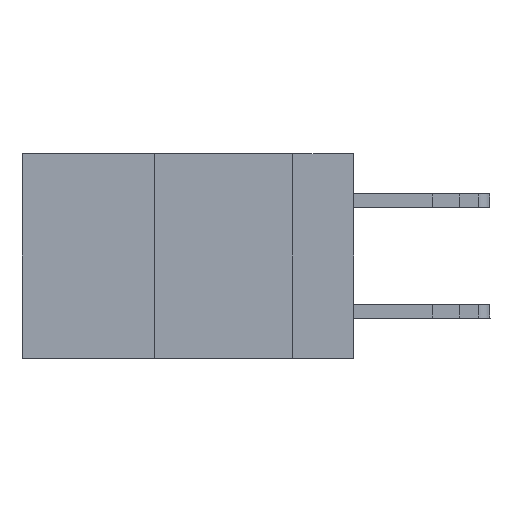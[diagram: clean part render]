
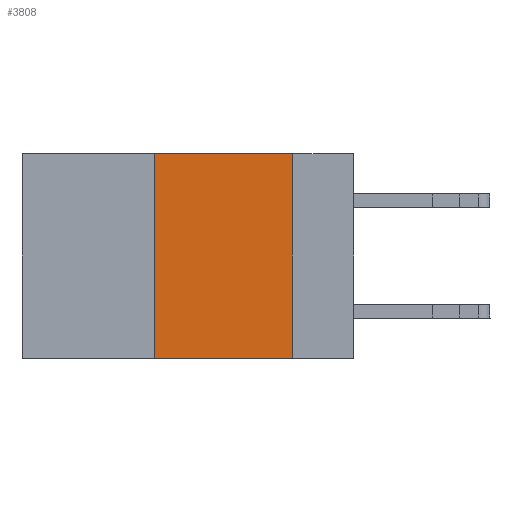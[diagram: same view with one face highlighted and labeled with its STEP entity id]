
A CAD part, left-side view. The second image highlights one B-rep face of the part: STEP entity #3808.
In plain terms, the highlighted planar face has unit normal (-1, 0, 0).
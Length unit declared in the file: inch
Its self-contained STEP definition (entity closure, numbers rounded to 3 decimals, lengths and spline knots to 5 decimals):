
#539 = FACE_OUTER_BOUND ( 'NONE', #1060, .T. ) ;
#824 = CARTESIAN_POINT ( 'NONE',  ( 0., 0.11, -0.37 ) ) ;
#966 = AXIS2_PLACEMENT_3D ( 'NONE', #1714, #16997, #7418 ) ;
#981 = VERTEX_POINT ( 'NONE', #6675 ) ;
#1012 = ORIENTED_EDGE ( 'NONE', *, *, #10371, .F. ) ;
#1060 = EDGE_LOOP ( 'NONE', ( #17634, #1012, #13462, #4346 ) ) ;
#1296 = LINE ( 'NONE', #4005, #12722 ) ;
#1714 = CARTESIAN_POINT ( 'NONE',  ( 0., 0.6, 0. ) ) ;
#2672 = DIRECTION ( 'NONE',  ( 0., -1., 0. ) ) ;
#2732 = EDGE_CURVE ( 'NONE', #981, #13722, #12860, .T. ) ;
#3287 = VECTOR ( 'NONE', #2672, 39.37008 ) ;
#3808 = ADVANCED_FACE ( 'NONE', ( #539 ), #10044, .F. ) ;
#4005 = CARTESIAN_POINT ( 'NONE',  ( 0., 0.11, 0. ) ) ;
#4219 = VERTEX_POINT ( 'NONE', #14077 ) ;
#4346 = ORIENTED_EDGE ( 'NONE', *, *, #14621, .T. ) ;
#5191 = LINE ( 'NONE', #17231, #6292 ) ;
#5352 = VERTEX_POINT ( 'NONE', #824 ) ;
#5564 = CARTESIAN_POINT ( 'NONE',  ( 0., 0.6, 0. ) ) ;
#6292 = VECTOR ( 'NONE', #9259, 39.37008 ) ;
#6675 = CARTESIAN_POINT ( 'NONE',  ( 0., 0.36, -0.37 ) ) ;
#7063 = CARTESIAN_POINT ( 'NONE',  ( 0., 0.36, 0. ) ) ;
#7418 = DIRECTION ( 'NONE',  ( 0., 0., -1. ) ) ;
#7817 = EDGE_CURVE ( 'NONE', #4219, #5352, #1296, .T. ) ;
#7864 = CARTESIAN_POINT ( 'NONE',  ( 0., 0.36, 0. ) ) ;
#8353 = DIRECTION ( 'NONE',  ( 0., 0., -1. ) ) ;
#9259 = DIRECTION ( 'NONE',  ( 0., -1., 0. ) ) ;
#10044 = PLANE ( 'NONE',  #966 ) ;
#10371 = EDGE_CURVE ( 'NONE', #13722, #4219, #12105, .T. ) ;
#10564 = VECTOR ( 'NONE', #12948, 39.37008 ) ;
#12105 = LINE ( 'NONE', #5564, #3287 ) ;
#12722 = VECTOR ( 'NONE', #8353, 39.37008 ) ;
#12860 = LINE ( 'NONE', #7063, #10564 ) ;
#12948 = DIRECTION ( 'NONE',  ( 0., 0., 1. ) ) ;
#13462 = ORIENTED_EDGE ( 'NONE', *, *, #2732, .F. ) ;
#13722 = VERTEX_POINT ( 'NONE', #7864 ) ;
#14077 = CARTESIAN_POINT ( 'NONE',  ( 0., 0.11, 0. ) ) ;
#14621 = EDGE_CURVE ( 'NONE', #981, #5352, #5191, .T. ) ;
#16997 = DIRECTION ( 'NONE',  ( 1., 0., 0. ) ) ;
#17231 = CARTESIAN_POINT ( 'NONE',  ( 0., 0.6, -0.37 ) ) ;
#17634 = ORIENTED_EDGE ( 'NONE', *, *, #7817, .F. ) ;
